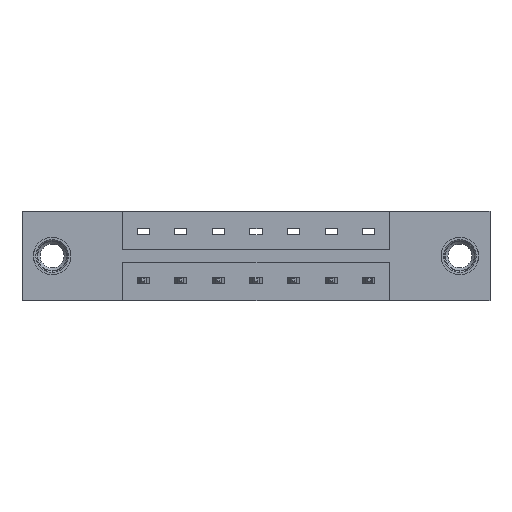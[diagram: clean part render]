
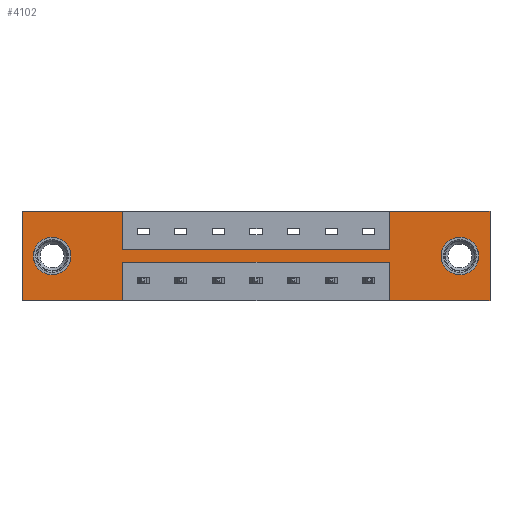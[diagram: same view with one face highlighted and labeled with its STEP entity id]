
A CAD part, front view. The second image highlights one B-rep face of the part: STEP entity #4102.
In plain terms, the highlighted planar face has unit normal (0, -1, 0).
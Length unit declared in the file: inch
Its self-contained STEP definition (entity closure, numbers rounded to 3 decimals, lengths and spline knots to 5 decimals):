
#51 = ORIENTED_EDGE ( 'NONE', *, *, #4986, .F. ) ;
#63 = VERTEX_POINT ( 'NONE', #1225 ) ;
#71 = VERTEX_POINT ( 'NONE', #5875 ) ;
#80 = CARTESIAN_POINT ( 'NONE',  ( 1.94, 0., 0. ) ) ;
#121 = CARTESIAN_POINT ( 'NONE',  ( 0.125, 0., -0.107 ) ) ;
#143 = CARTESIAN_POINT ( 'NONE',  ( 1.815, 0., -0.185 ) ) ;
#191 = CARTESIAN_POINT ( 'NONE',  ( 0.125, 0., -0.263 ) ) ;
#199 = EDGE_CURVE ( 'NONE', #5350, #63, #3484, .T. ) ;
#288 = ORIENTED_EDGE ( 'NONE', *, *, #8342, .T. ) ;
#354 = LINE ( 'NONE', #2717, #7722 ) ;
#445 = CARTESIAN_POINT ( 'NONE',  ( 1.5225, 0., -0.2115 ) ) ;
#679 = ORIENTED_EDGE ( 'NONE', *, *, #8528, .F. ) ;
#736 = ORIENTED_EDGE ( 'NONE', *, *, #1278, .F. ) ;
#763 = AXIS2_PLACEMENT_3D ( 'NONE', #5695, #9609, #1807 ) ;
#836 = DIRECTION ( 'NONE',  ( 1., 0., 0. ) ) ;
#860 = DIRECTION ( 'NONE',  ( 0., 0., 1. ) ) ;
#863 = DIRECTION ( 'NONE',  ( 0., 0., -1. ) ) ;
#916 = CIRCLE ( 'NONE', #763, 0.078 ) ;
#1130 = ORIENTED_EDGE ( 'NONE', *, *, #8823, .T. ) ;
#1225 = CARTESIAN_POINT ( 'NONE',  ( 0., 0., -0.37 ) ) ;
#1278 = EDGE_CURVE ( 'NONE', #4582, #2570, #7974, .T. ) ;
#1337 = EDGE_CURVE ( 'NONE', #6441, #2222, #8595, .T. ) ;
#1643 = CARTESIAN_POINT ( 'NONE',  ( 0.4175, 0., -0.1585 ) ) ;
#1684 = LINE ( 'NONE', #8525, #9323 ) ;
#1769 = DIRECTION ( 'NONE',  ( 0., 1., 0. ) ) ;
#1807 = DIRECTION ( 'NONE',  ( 0., 0., -1. ) ) ;
#1837 = VERTEX_POINT ( 'NONE', #3375 ) ;
#1895 = EDGE_CURVE ( 'NONE', #6491, #8865, #6961, .T. ) ;
#1950 = AXIS2_PLACEMENT_3D ( 'NONE', #5816, #5911, #2917 ) ;
#1965 = ORIENTED_EDGE ( 'NONE', *, *, #7212, .F. ) ;
#1987 = ORIENTED_EDGE ( 'NONE', *, *, #1337, .F. ) ;
#2055 = ORIENTED_EDGE ( 'NONE', *, *, #7959, .F. ) ;
#2166 = LINE ( 'NONE', #5211, #8402 ) ;
#2221 = CIRCLE ( 'NONE', #6252, 0.078 ) ;
#2222 = VERTEX_POINT ( 'NONE', #5544 ) ;
#2415 = DIRECTION ( 'NONE',  ( 0., 1., 0. ) ) ;
#2463 = DIRECTION ( 'NONE',  ( 0., 0., -1. ) ) ;
#2562 = EDGE_CURVE ( 'NONE', #4700, #71, #8399, .T. ) ;
#2570 = VERTEX_POINT ( 'NONE', #6158 ) ;
#2623 = VECTOR ( 'NONE', #6688, 39.37008 ) ;
#2717 = CARTESIAN_POINT ( 'NONE',  ( 1.5225, 0., -0.2115 ) ) ;
#2759 = VECTOR ( 'NONE', #3054, 39.37008 ) ;
#2917 = DIRECTION ( 'NONE',  ( 0., 0., 1. ) ) ;
#3001 = ORIENTED_EDGE ( 'NONE', *, *, #3482, .F. ) ;
#3054 = DIRECTION ( 'NONE',  ( 0., 0., -1. ) ) ;
#3128 = EDGE_LOOP ( 'NONE', ( #288, #9532 ) ) ;
#3330 = CARTESIAN_POINT ( 'NONE',  ( 0.4175, 0., -0.2115 ) ) ;
#3331 = VECTOR ( 'NONE', #3806, 39.37008 ) ;
#3375 = CARTESIAN_POINT ( 'NONE',  ( 1.815, 0., -0.263 ) ) ;
#3388 = VERTEX_POINT ( 'NONE', #6892 ) ;
#3399 = CARTESIAN_POINT ( 'NONE',  ( 0.4175, 0., -0.37 ) ) ;
#3482 = EDGE_CURVE ( 'NONE', #2570, #6441, #6372, .T. ) ;
#3484 = LINE ( 'NONE', #3539, #5450 ) ;
#3539 = CARTESIAN_POINT ( 'NONE',  ( 0., 0., -0.37 ) ) ;
#3584 = VECTOR ( 'NONE', #2463, 39.37008 ) ;
#3618 = CARTESIAN_POINT ( 'NONE',  ( 0., 0., 0. ) ) ;
#3774 = DIRECTION ( 'NONE',  ( 0., 0., 1. ) ) ;
#3806 = DIRECTION ( 'NONE',  ( 0., 0., -1. ) ) ;
#3989 = ORIENTED_EDGE ( 'NONE', *, *, #199, .F. ) ;
#4102 = ADVANCED_FACE ( 'NONE', ( #8907, #9713, #6654 ), #7465, .T. ) ;
#4163 = CIRCLE ( 'NONE', #8548, 0.078 ) ;
#4244 = CARTESIAN_POINT ( 'NONE',  ( 0.4175, 0., -0.2115 ) ) ;
#4269 = EDGE_LOOP ( 'NONE', ( #4304, #1130 ) ) ;
#4304 = ORIENTED_EDGE ( 'NONE', *, *, #1895, .T. ) ;
#4439 = EDGE_CURVE ( 'NONE', #3388, #6225, #354, .T. ) ;
#4529 = EDGE_CURVE ( 'NONE', #2222, #5026, #2166, .T. ) ;
#4582 = VERTEX_POINT ( 'NONE', #7542 ) ;
#4700 = VERTEX_POINT ( 'NONE', #80 ) ;
#4745 = CARTESIAN_POINT ( 'NONE',  ( 0.125, 0., -0.185 ) ) ;
#4753 = DIRECTION ( 'NONE',  ( -1., 0., 0. ) ) ;
#4768 = ORIENTED_EDGE ( 'NONE', *, *, #4529, .F. ) ;
#4986 = EDGE_CURVE ( 'NONE', #63, #4582, #9122, .T. ) ;
#5024 = DIRECTION ( 'NONE',  ( -1., 0., 0. ) ) ;
#5026 = VERTEX_POINT ( 'NONE', #9879 ) ;
#5042 = DIRECTION ( 'NONE',  ( 0., -1., 0. ) ) ;
#5107 = CARTESIAN_POINT ( 'NONE',  ( 1.815, 0., -0.107 ) ) ;
#5211 = CARTESIAN_POINT ( 'NONE',  ( 1.5225, 0., -0.1585 ) ) ;
#5350 = VERTEX_POINT ( 'NONE', #3399 ) ;
#5450 = VECTOR ( 'NONE', #5024, 39.37008 ) ;
#5454 = VECTOR ( 'NONE', #4753, 39.37008 ) ;
#5544 = CARTESIAN_POINT ( 'NONE',  ( 1.5225, 0., -0.1585 ) ) ;
#5695 = CARTESIAN_POINT ( 'NONE',  ( 1.815, 0., -0.185 ) ) ;
#5707 = EDGE_CURVE ( 'NONE', #71, #3388, #8824, .T. ) ;
#5816 = CARTESIAN_POINT ( 'NONE',  ( 0.125, 0., -0.185 ) ) ;
#5868 = AXIS2_PLACEMENT_3D ( 'NONE', #5939, #5042, #8138 ) ;
#5870 = CARTESIAN_POINT ( 'NONE',  ( 0., 0., -0.37 ) ) ;
#5875 = CARTESIAN_POINT ( 'NONE',  ( 1.94, 0., -0.37 ) ) ;
#5911 = DIRECTION ( 'NONE',  ( 0., 1., 0. ) ) ;
#5939 = CARTESIAN_POINT ( 'NONE',  ( 0., 0., -0.37 ) ) ;
#5962 = DIRECTION ( 'NONE',  ( 0., 0., 1. ) ) ;
#6137 = VERTEX_POINT ( 'NONE', #5107 ) ;
#6158 = CARTESIAN_POINT ( 'NONE',  ( 0.4175, 0., 0. ) ) ;
#6192 = VERTEX_POINT ( 'NONE', #4244 ) ;
#6225 = VERTEX_POINT ( 'NONE', #445 ) ;
#6252 = AXIS2_PLACEMENT_3D ( 'NONE', #4745, #1769, #860 ) ;
#6372 = LINE ( 'NONE', #7906, #3584 ) ;
#6441 = VERTEX_POINT ( 'NONE', #9409 ) ;
#6491 = VERTEX_POINT ( 'NONE', #121 ) ;
#6654 = FACE_OUTER_BOUND ( 'NONE', #9084, .T. ) ;
#6688 = DIRECTION ( 'NONE',  ( -1., 0., 0. ) ) ;
#6892 = CARTESIAN_POINT ( 'NONE',  ( 1.5225, 0., -0.37 ) ) ;
#6942 = VECTOR ( 'NONE', #7770, 39.37008 ) ;
#6961 = CIRCLE ( 'NONE', #1950, 0.078 ) ;
#6990 = DIRECTION ( 'NONE',  ( 1., 0., 0. ) ) ;
#7212 = EDGE_CURVE ( 'NONE', #5026, #4700, #1684, .T. ) ;
#7436 = VECTOR ( 'NONE', #836, 39.37008 ) ;
#7465 = PLANE ( 'NONE',  #5868 ) ;
#7542 = CARTESIAN_POINT ( 'NONE',  ( 0., 0., 0. ) ) ;
#7623 = LINE ( 'NONE', #9967, #3331 ) ;
#7722 = VECTOR ( 'NONE', #9784, 39.37008 ) ;
#7770 = DIRECTION ( 'NONE',  ( 1., 0., 0. ) ) ;
#7869 = CARTESIAN_POINT ( 'NONE',  ( 0., 0., 0. ) ) ;
#7906 = CARTESIAN_POINT ( 'NONE',  ( 0.4175, 0., -0.1585 ) ) ;
#7959 = EDGE_CURVE ( 'NONE', #6192, #5350, #7623, .T. ) ;
#7974 = LINE ( 'NONE', #7869, #6942 ) ;
#8138 = DIRECTION ( 'NONE',  ( 0., 0., -1. ) ) ;
#8279 = ORIENTED_EDGE ( 'NONE', *, *, #4439, .F. ) ;
#8342 = EDGE_CURVE ( 'NONE', #6137, #1837, #4163, .T. ) ;
#8399 = LINE ( 'NONE', #10026, #2759 ) ;
#8402 = VECTOR ( 'NONE', #3774, 39.37008 ) ;
#8519 = ORIENTED_EDGE ( 'NONE', *, *, #2562, .F. ) ;
#8525 = CARTESIAN_POINT ( 'NONE',  ( 0., 0., 0. ) ) ;
#8528 = EDGE_CURVE ( 'NONE', #6225, #6192, #9535, .T. ) ;
#8548 = AXIS2_PLACEMENT_3D ( 'NONE', #143, #2415, #863 ) ;
#8595 = LINE ( 'NONE', #1643, #7436 ) ;
#8823 = EDGE_CURVE ( 'NONE', #8865, #6491, #2221, .T. ) ;
#8824 = LINE ( 'NONE', #5870, #2623 ) ;
#8865 = VERTEX_POINT ( 'NONE', #191 ) ;
#8907 = FACE_BOUND ( 'NONE', #3128, .T. ) ;
#9084 = EDGE_LOOP ( 'NONE', ( #8279, #9452, #8519, #1965, #4768, #1987, #3001, #736, #51, #3989, #2055, #679 ) ) ;
#9122 = LINE ( 'NONE', #3618, #9362 ) ;
#9323 = VECTOR ( 'NONE', #6990, 39.37008 ) ;
#9362 = VECTOR ( 'NONE', #5962, 39.37008 ) ;
#9396 = EDGE_CURVE ( 'NONE', #1837, #6137, #916, .T. ) ;
#9409 = CARTESIAN_POINT ( 'NONE',  ( 0.4175, 0., -0.1585 ) ) ;
#9452 = ORIENTED_EDGE ( 'NONE', *, *, #5707, .F. ) ;
#9532 = ORIENTED_EDGE ( 'NONE', *, *, #9396, .T. ) ;
#9535 = LINE ( 'NONE', #3330, #5454 ) ;
#9609 = DIRECTION ( 'NONE',  ( 0., 1., 0. ) ) ;
#9713 = FACE_BOUND ( 'NONE', #4269, .T. ) ;
#9784 = DIRECTION ( 'NONE',  ( 0., 0., 1. ) ) ;
#9879 = CARTESIAN_POINT ( 'NONE',  ( 1.5225, 0., 0. ) ) ;
#9967 = CARTESIAN_POINT ( 'NONE',  ( 0.4175, 0., -0.2115 ) ) ;
#10026 = CARTESIAN_POINT ( 'NONE',  ( 1.94, 0., 0. ) ) ;
